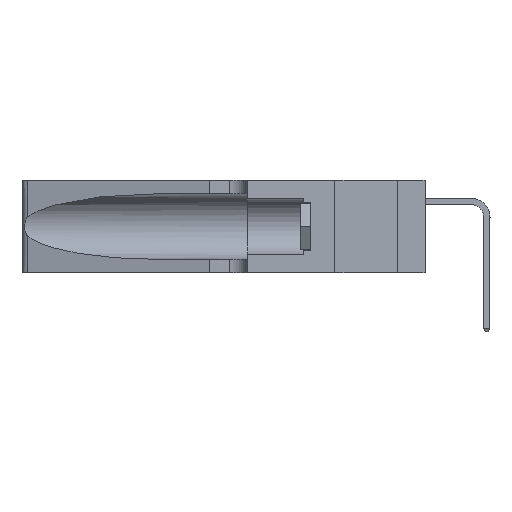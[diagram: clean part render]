
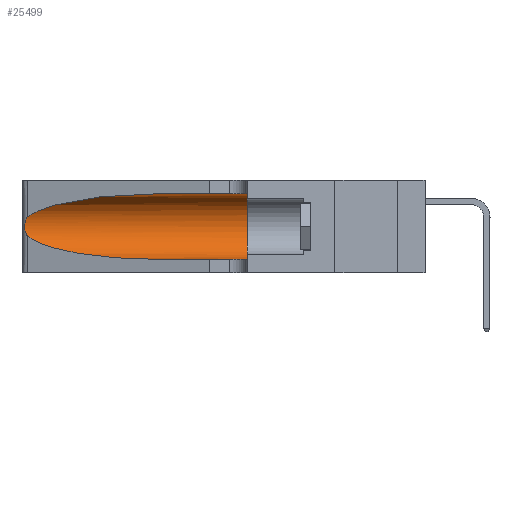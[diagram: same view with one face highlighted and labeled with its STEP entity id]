
A CAD part, left-side view. The second image highlights one B-rep face of the part: STEP entity #25499.
In plain terms, the highlighted cylindrical face has radius 3.308 mm (diameter 6.617 mm), a partial arc.
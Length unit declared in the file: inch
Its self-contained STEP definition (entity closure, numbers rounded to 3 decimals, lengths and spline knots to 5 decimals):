
#207 = B_SPLINE_CURVE_WITH_KNOTS ( 'NONE', 3,
 ( #26613, #29606, #32633, #14680, #35644, #17704, #38607, #20739, #2714, #23752, #5738, #26743, #8769, #29736 ),
 .UNSPECIFIED., .F., .F.,
 ( 4, 2, 2, 2, 2, 2, 4 ),
 ( 0., 0.00027, 0.00053, 0.00107, 0.0016, 0.00187, 0.00214 ),
 .UNSPECIFIED. ) ;
#1416 = DIRECTION ( 'NONE',  ( 0., 0., -1. ) ) ;
#2482 = CARTESIAN_POINT ( 'NONE',  ( 0.1305, 0.72297, 0.31525 ) ) ;
#2714 = CARTESIAN_POINT ( 'NONE',  ( 0.26017, 1.23833, 0.17102 ) ) ;
#3336 = CYLINDRICAL_SURFACE ( 'NONE', #30837, 0.13025 ) ;
#5220 = VECTOR ( 'NONE', #11863, 39.37008 ) ;
#5738 = CARTESIAN_POINT ( 'NONE',  ( 0.25789, 1.23486, 0.15765 ) ) ;
#6189 = LINE ( 'NONE', #8819, #5220 ) ;
#6548 = CARTESIAN_POINT ( 'NONE',  ( 0.25487, 1.22718, 0.14631 ) ) ;
#6760 = ORIENTED_EDGE ( 'NONE', *, *, #35984, .T. ) ;
#7545 = CARTESIAN_POINT ( 'NONE',  ( 0.1305, 0.35, 0.31525 ) ) ;
#8743 = CARTESIAN_POINT ( 'NONE',  ( 0.1305, 0.72297, 0.31525 ) ) ;
#8769 = CARTESIAN_POINT ( 'NONE',  ( 0.25555, 1.22993, 0.14849 ) ) ;
#8819 = CARTESIAN_POINT ( 'NONE',  ( 0.1305, 1.61858, 0.31525 ) ) ;
#10459 = LINE ( 'NONE', #11454, #27360 ) ;
#11454 = CARTESIAN_POINT ( 'NONE',  ( 0.1305, 1.61858, 0.05475 ) ) ;
#11863 = DIRECTION ( 'NONE',  ( 0., -1., 0. ) ) ;
#12622 = CARTESIAN_POINT ( 'NONE',  ( 0.1305, 0.72297, 0.05475 ) ) ;
#13568 = DIRECTION ( 'NONE',  ( 0., 1., 0. ) ) ;
#14539 = ORIENTED_EDGE ( 'NONE', *, *, #22863, .F. ) ;
#14680 = CARTESIAN_POINT ( 'NONE',  ( 0.25787, 1.23484, 0.2124 ) ) ;
#16459 = EDGE_CURVE ( 'NONE', #26443, #35963, #32993, .T. ) ;
#17473 = CARTESIAN_POINT ( 'NONE',  ( 0.2373, 1.15595, 0.28018 ) ) ;
#17704 = CARTESIAN_POINT ( 'NONE',  ( 0.26018, 1.23835, 0.19895 ) ) ;
#19473 = DIRECTION ( 'NONE',  ( 0., -1., 0. ) ) ;
#20380 = DIRECTION ( 'NONE',  ( 0., -1., 0. ) ) ;
#20506 = CARTESIAN_POINT ( 'NONE',  ( 0.18966, 0.96281, 0.31525 ) ) ;
#20703 = CARTESIAN_POINT ( 'NONE',  ( 0.25487, 1.22718, 0.14631 ) ) ;
#20739 = CARTESIAN_POINT ( 'NONE',  ( 0.26075, 1.23896, 0.178 ) ) ;
#20840 = VERTEX_POINT ( 'NONE', #36352 ) ;
#22591 = VERTEX_POINT ( 'NONE', #7545 ) ;
#22725 = VERTEX_POINT ( 'NONE', #26135 ) ;
#22782 = EDGE_CURVE ( 'NONE', #22725, #20840, #10459, .T. ) ;
#22863 = EDGE_CURVE ( 'NONE', #26443, #22591, #6189, .T. ) ;
#23451 = EDGE_CURVE ( 'NONE', #35963, #32118, #207, .T. ) ;
#23532 = CARTESIAN_POINT ( 'NONE',  ( 0.25487, 1.22718, 0.22369 ) ) ;
#23752 = CARTESIAN_POINT ( 'NONE',  ( 0.25856, 1.23593, 0.16098 ) ) ;
#24449 = ORIENTED_EDGE ( 'NONE', *, *, #23451, .T. ) ;
#24548 = CARTESIAN_POINT ( 'NONE',  ( 0.2373, 1.15595, 0.08982 ) ) ;
#25499 = ADVANCED_FACE ( 'NONE', ( #35237 ), #3336, .F. ) ;
#25695 =( BOUNDED_CURVE ( )  B_SPLINE_CURVE ( 3, ( #6548, #24548, #30552, #12622 ),
 .UNSPECIFIED., .F., .T. ) 
 B_SPLINE_CURVE_WITH_KNOTS ( ( 4, 4 ),
 ( 3.44316, 4.71239 ),
 .UNSPECIFIED. ) 
 CURVE ( )  GEOMETRIC_REPRESENTATION_ITEM ( )  RATIONAL_B_SPLINE_CURVE ( ( 1., 0.87, 0.87, 1. ) ) 
 REPRESENTATION_ITEM ( '' )  );
#25987 = ORIENTED_EDGE ( 'NONE', *, *, #16459, .T. ) ;
#26135 = CARTESIAN_POINT ( 'NONE',  ( 0.1305, 0.72297, 0.05475 ) ) ;
#26443 = VERTEX_POINT ( 'NONE', #8743 ) ;
#26613 = CARTESIAN_POINT ( 'NONE',  ( 0.25487, 1.22718, 0.22369 ) ) ;
#26743 = CARTESIAN_POINT ( 'NONE',  ( 0.25639, 1.23186, 0.15144 ) ) ;
#27270 = ORIENTED_EDGE ( 'NONE', *, *, #22782, .T. ) ;
#27360 = VECTOR ( 'NONE', #20380, 39.37008 ) ;
#27564 = CIRCLE ( 'NONE', #31655, 0.13025 ) ;
#29596 = EDGE_LOOP ( 'NONE', ( #25987, #24449, #6760, #27270, #29789, #14539 ) ) ;
#29606 = CARTESIAN_POINT ( 'NONE',  ( 0.25555, 1.22994, 0.2215 ) ) ;
#29736 = CARTESIAN_POINT ( 'NONE',  ( 0.25487, 1.22718, 0.14631 ) ) ;
#29789 = ORIENTED_EDGE ( 'NONE', *, *, #33011, .F. ) ;
#30552 = CARTESIAN_POINT ( 'NONE',  ( 0.18966, 0.96281, 0.05475 ) ) ;
#30837 = AXIS2_PLACEMENT_3D ( 'NONE', #37271, #19473, #1416 ) ;
#31518 = CARTESIAN_POINT ( 'NONE',  ( 0.1305, 0.35, 0.185 ) ) ;
#31655 = AXIS2_PLACEMENT_3D ( 'NONE', #31518, #13568, #34515 ) ;
#32118 = VERTEX_POINT ( 'NONE', #20703 ) ;
#32633 = CARTESIAN_POINT ( 'NONE',  ( 0.25639, 1.23184, 0.21858 ) ) ;
#32993 =( BOUNDED_CURVE ( )  B_SPLINE_CURVE ( 3, ( #2482, #20506, #17473, #23532 ),
 .UNSPECIFIED., .F., .F. ) 
 B_SPLINE_CURVE_WITH_KNOTS ( ( 4, 4 ),
 ( 1.5708, 2.84003 ),
 .UNSPECIFIED. ) 
 CURVE ( )  GEOMETRIC_REPRESENTATION_ITEM ( )  RATIONAL_B_SPLINE_CURVE ( ( 1., 0.87, 0.87, 1. ) ) 
 REPRESENTATION_ITEM ( '' )  );
#33011 = EDGE_CURVE ( 'NONE', #22591, #20840, #27564, .T. ) ;
#34515 = DIRECTION ( 'NONE',  ( 0., 0., 1. ) ) ;
#35237 = FACE_OUTER_BOUND ( 'NONE', #29596, .T. ) ;
#35644 = CARTESIAN_POINT ( 'NONE',  ( 0.25854, 1.2359, 0.20912 ) ) ;
#35963 = VERTEX_POINT ( 'NONE', #36440 ) ;
#35984 = EDGE_CURVE ( 'NONE', #32118, #22725, #25695, .T. ) ;
#36352 = CARTESIAN_POINT ( 'NONE',  ( 0.1305, 0.35, 0.05475 ) ) ;
#36440 = CARTESIAN_POINT ( 'NONE',  ( 0.25487, 1.22718, 0.22369 ) ) ;
#37271 = CARTESIAN_POINT ( 'NONE',  ( 0.1305, 1.61858, 0.185 ) ) ;
#38607 = CARTESIAN_POINT ( 'NONE',  ( 0.26075, 1.23896, 0.19203 ) ) ;
